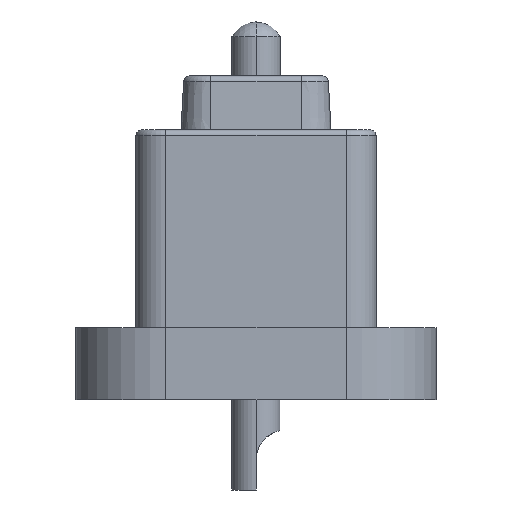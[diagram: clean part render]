
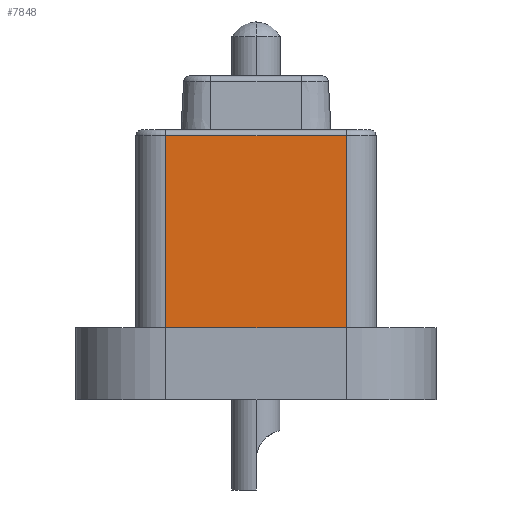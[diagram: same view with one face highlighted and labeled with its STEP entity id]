
A CAD part, left-side view. The second image highlights one B-rep face of the part: STEP entity #7848.
In plain terms, the highlighted planar face has unit normal (-1, 0, 0).
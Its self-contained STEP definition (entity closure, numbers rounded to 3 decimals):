
#112 = DIRECTION ( 'NONE',  ( 0., 1., 0. ) ) ;
#223 = CARTESIAN_POINT ( 'NONE',  ( -8.45, 1.5, -3.3 ) ) ;
#400 = DIRECTION ( 'NONE',  ( 0., 0., 1. ) ) ;
#752 = PLANE ( 'NONE',  #4876 ) ;
#1139 = ORIENTED_EDGE ( 'NONE', *, *, #3902, .T. ) ;
#1157 = VECTOR ( 'NONE', #4211, 1000. ) ;
#1600 = CARTESIAN_POINT ( 'NONE',  ( -8.45, 1.5, -0.1 ) ) ;
#1807 = ORIENTED_EDGE ( 'NONE', *, *, #7494, .T. ) ;
#2145 = LINE ( 'NONE', #4747, #4870 ) ;
#2343 = LINE ( 'NONE', #4945, #5819 ) ;
#2605 = CARTESIAN_POINT ( 'NONE',  ( -8.45, 1.5, -0.1 ) ) ;
#3352 = CARTESIAN_POINT ( 'NONE',  ( -8.45, 0., -1.7 ) ) ;
#3534 = EDGE_LOOP ( 'NONE', ( #7752, #1807, #7340, #1139 ) ) ;
#3637 = LINE ( 'NONE', #6241, #8307 ) ;
#3902 = EDGE_CURVE ( 'NONE', #5338, #5098, #2343, .T. ) ;
#4211 = DIRECTION ( 'NONE',  ( 0., 0., -1. ) ) ;
#4380 = EDGE_CURVE ( 'NONE', #5098, #6545, #7454, .T. ) ;
#4701 = CARTESIAN_POINT ( 'NONE',  ( -8.45, -1.5, -3.3 ) ) ;
#4747 = CARTESIAN_POINT ( 'NONE',  ( -8.45, 1.5, -3.3 ) ) ;
#4870 = VECTOR ( 'NONE', #7365, 1000. ) ;
#4876 = AXIS2_PLACEMENT_3D ( 'NONE', #3352, #5954, #112 ) ;
#4945 = CARTESIAN_POINT ( 'NONE',  ( -8.45, -1.5, -0.1 ) ) ;
#5098 = VERTEX_POINT ( 'NONE', #2605 ) ;
#5338 = VERTEX_POINT ( 'NONE', #5655 ) ;
#5655 = CARTESIAN_POINT ( 'NONE',  ( -8.45, -1.5, -0.1 ) ) ;
#5819 = VECTOR ( 'NONE', #7558, 1000. ) ;
#5954 = DIRECTION ( 'NONE',  ( 1., 0., 0. ) ) ;
#6241 = CARTESIAN_POINT ( 'NONE',  ( -8.45, -1.5, -3.3 ) ) ;
#6545 = VERTEX_POINT ( 'NONE', #223 ) ;
#6598 = FACE_OUTER_BOUND ( 'NONE', #3534, .T. ) ;
#7340 = ORIENTED_EDGE ( 'NONE', *, *, #8398, .T. ) ;
#7365 = DIRECTION ( 'NONE',  ( 0., -1., 0. ) ) ;
#7454 = LINE ( 'NONE', #1600, #1157 ) ;
#7494 = EDGE_CURVE ( 'NONE', #6545, #8200, #2145, .T. ) ;
#7558 = DIRECTION ( 'NONE',  ( 0., 1., 0. ) ) ;
#7752 = ORIENTED_EDGE ( 'NONE', *, *, #4380, .T. ) ;
#7848 = ADVANCED_FACE ( 'NONE', ( #6598 ), #752, .F. ) ;
#8200 = VERTEX_POINT ( 'NONE', #4701 ) ;
#8307 = VECTOR ( 'NONE', #400, 1000. ) ;
#8398 = EDGE_CURVE ( 'NONE', #8200, #5338, #3637, .T. ) ;
